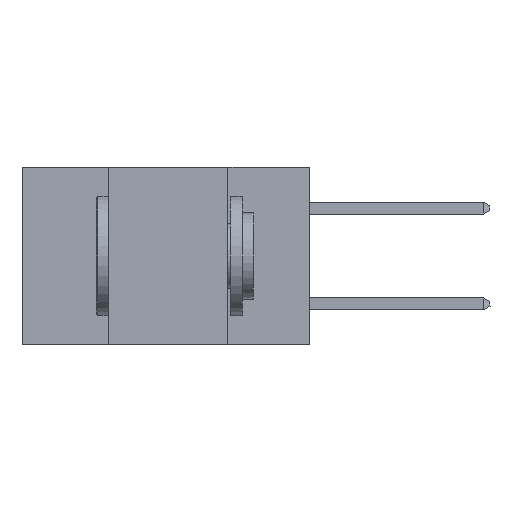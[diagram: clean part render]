
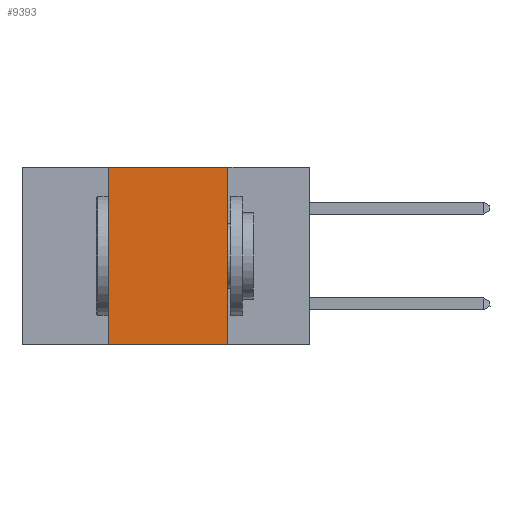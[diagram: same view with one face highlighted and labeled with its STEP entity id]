
A CAD part, left-side view. The second image highlights one B-rep face of the part: STEP entity #9393.
In plain terms, the highlighted planar face has unit normal (-1, 0, 0).
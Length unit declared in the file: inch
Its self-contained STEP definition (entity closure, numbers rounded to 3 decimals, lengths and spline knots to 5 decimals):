
#24 = CARTESIAN_POINT ( 'NONE',  ( 0., 0.17, -0.37 ) ) ;
#144 = CARTESIAN_POINT ( 'NONE',  ( 0., 0.17, 0. ) ) ;
#145 = FACE_OUTER_BOUND ( 'NONE', #16389, .T. ) ;
#387 = CARTESIAN_POINT ( 'NONE',  ( 0., 0.42, 0. ) ) ;
#1989 = EDGE_CURVE ( 'NONE', #11924, #17976, #19439, .T. ) ;
#3261 = DIRECTION ( 'NONE',  ( 1., 0., 0. ) ) ;
#3458 = EDGE_CURVE ( 'NONE', #18335, #6597, #5120, .T. ) ;
#4045 = CARTESIAN_POINT ( 'NONE',  ( 0., 0.17, 0. ) ) ;
#4840 = ORIENTED_EDGE ( 'NONE', *, *, #3458, .F. ) ;
#5120 = LINE ( 'NONE', #7492, #9023 ) ;
#5492 = ORIENTED_EDGE ( 'NONE', *, *, #9016, .F. ) ;
#5669 = DIRECTION ( 'NONE',  ( 0., 0., -1. ) ) ;
#5698 = LINE ( 'NONE', #387, #10082 ) ;
#6274 = LINE ( 'NONE', #4045, #14360 ) ;
#6597 = VERTEX_POINT ( 'NONE', #144 ) ;
#7492 = CARTESIAN_POINT ( 'NONE',  ( 0., 0.6, 0. ) ) ;
#8744 = DIRECTION ( 'NONE',  ( 0., -1., 0. ) ) ;
#9016 = EDGE_CURVE ( 'NONE', #6597, #17976, #6274, .T. ) ;
#9023 = VECTOR ( 'NONE', #8744, 39.37008 ) ;
#9393 = ADVANCED_FACE ( 'NONE', ( #145 ), #13914, .F. ) ;
#9488 = CARTESIAN_POINT ( 'NONE',  ( 0., 0.6, -0.37 ) ) ;
#10082 = VECTOR ( 'NONE', #18059, 39.37008 ) ;
#11043 = AXIS2_PLACEMENT_3D ( 'NONE', #12994, #3261, #14561 ) ;
#11594 = CARTESIAN_POINT ( 'NONE',  ( 0., 0.42, -0.37 ) ) ;
#11924 = VERTEX_POINT ( 'NONE', #11594 ) ;
#12994 = CARTESIAN_POINT ( 'NONE',  ( 0., 0.6, 0. ) ) ;
#13914 = PLANE ( 'NONE',  #11043 ) ;
#14360 = VECTOR ( 'NONE', #5669, 39.37008 ) ;
#14561 = DIRECTION ( 'NONE',  ( 0., 0., -1. ) ) ;
#15200 = ORIENTED_EDGE ( 'NONE', *, *, #1989, .T. ) ;
#15271 = VECTOR ( 'NONE', #16455, 39.37008 ) ;
#15419 = CARTESIAN_POINT ( 'NONE',  ( 0., 0.42, 0. ) ) ;
#16389 = EDGE_LOOP ( 'NONE', ( #5492, #4840, #19601, #15200 ) ) ;
#16455 = DIRECTION ( 'NONE',  ( 0., -1., 0. ) ) ;
#17976 = VERTEX_POINT ( 'NONE', #24 ) ;
#18059 = DIRECTION ( 'NONE',  ( 0., 0., 1. ) ) ;
#18335 = VERTEX_POINT ( 'NONE', #15419 ) ;
#19439 = LINE ( 'NONE', #9488, #15271 ) ;
#19601 = ORIENTED_EDGE ( 'NONE', *, *, #19981, .F. ) ;
#19981 = EDGE_CURVE ( 'NONE', #11924, #18335, #5698, .T. ) ;
